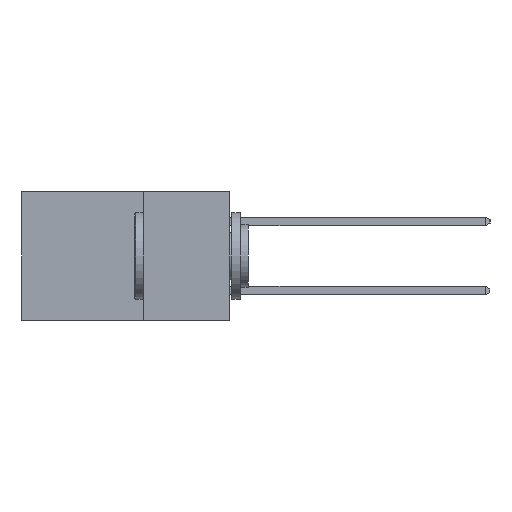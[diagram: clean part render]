
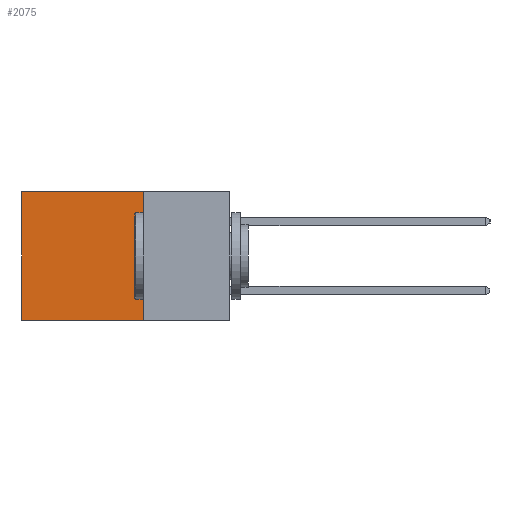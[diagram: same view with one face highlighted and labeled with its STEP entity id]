
A CAD part, left-side view. The second image highlights one B-rep face of the part: STEP entity #2075.
In plain terms, the highlighted planar face has unit normal (-1, 0, 0).
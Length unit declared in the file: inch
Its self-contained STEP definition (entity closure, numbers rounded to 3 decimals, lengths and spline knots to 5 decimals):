
#726 = VECTOR ( 'NONE', #13437, 39.37008 ) ;
#947 = CARTESIAN_POINT ( 'NONE',  ( 0.298, 0.25, -0.37 ) ) ;
#1084 = CARTESIAN_POINT ( 'NONE',  ( 0.298, 0.6, 0. ) ) ;
#1626 = EDGE_CURVE ( 'NONE', #5323, #4395, #10473, .T. ) ;
#1653 = CARTESIAN_POINT ( 'NONE',  ( 0.298, 0.25, -0.37 ) ) ;
#2075 = ADVANCED_FACE ( 'NONE', ( #10060 ), #10993, .F. ) ;
#3229 = LINE ( 'NONE', #14945, #12930 ) ;
#3589 = EDGE_CURVE ( 'NONE', #15904, #12487, #3229, .T. ) ;
#4163 = VECTOR ( 'NONE', #12348, 39.37008 ) ;
#4292 = CARTESIAN_POINT ( 'NONE',  ( 0.298, 0.6, -0.37 ) ) ;
#4395 = VERTEX_POINT ( 'NONE', #4292 ) ;
#5323 = VERTEX_POINT ( 'NONE', #947 ) ;
#5476 = CARTESIAN_POINT ( 'NONE',  ( 0.298, 0.25, 0. ) ) ;
#5817 = ORIENTED_EDGE ( 'NONE', *, *, #9772, .T. ) ;
#5913 = ORIENTED_EDGE ( 'NONE', *, *, #3589, .T. ) ;
#6612 = AXIS2_PLACEMENT_3D ( 'NONE', #9650, #16229, #14202 ) ;
#6769 = DIRECTION ( 'NONE',  ( 0., 0., -1. ) ) ;
#6845 = EDGE_LOOP ( 'NONE', ( #5817, #10048, #13834, #5913 ) ) ;
#7274 = CARTESIAN_POINT ( 'NONE',  ( 0.298, 0.6, 0. ) ) ;
#7565 = LINE ( 'NONE', #7274, #4163 ) ;
#9017 = CARTESIAN_POINT ( 'NONE',  ( 0.298, 0.25, 0. ) ) ;
#9650 = CARTESIAN_POINT ( 'NONE',  ( 0.298, 0.25, 0. ) ) ;
#9772 = EDGE_CURVE ( 'NONE', #12487, #4395, #7565, .T. ) ;
#10048 = ORIENTED_EDGE ( 'NONE', *, *, #1626, .F. ) ;
#10060 = FACE_OUTER_BOUND ( 'NONE', #6845, .T. ) ;
#10473 = LINE ( 'NONE', #1653, #726 ) ;
#10993 = PLANE ( 'NONE',  #6612 ) ;
#12047 = VECTOR ( 'NONE', #6769, 39.37008 ) ;
#12138 = EDGE_CURVE ( 'NONE', #15904, #5323, #12436, .T. ) ;
#12348 = DIRECTION ( 'NONE',  ( 0., 0., -1. ) ) ;
#12436 = LINE ( 'NONE', #5476, #12047 ) ;
#12487 = VERTEX_POINT ( 'NONE', #1084 ) ;
#12930 = VECTOR ( 'NONE', #13656, 39.37008 ) ;
#13437 = DIRECTION ( 'NONE',  ( 0., 1., 0. ) ) ;
#13656 = DIRECTION ( 'NONE',  ( 0., 1., 0. ) ) ;
#13834 = ORIENTED_EDGE ( 'NONE', *, *, #12138, .F. ) ;
#14202 = DIRECTION ( 'NONE',  ( 0., 0., -1. ) ) ;
#14945 = CARTESIAN_POINT ( 'NONE',  ( 0.298, 0.25, 0. ) ) ;
#15904 = VERTEX_POINT ( 'NONE', #9017 ) ;
#16229 = DIRECTION ( 'NONE',  ( 1., 0., 0. ) ) ;
